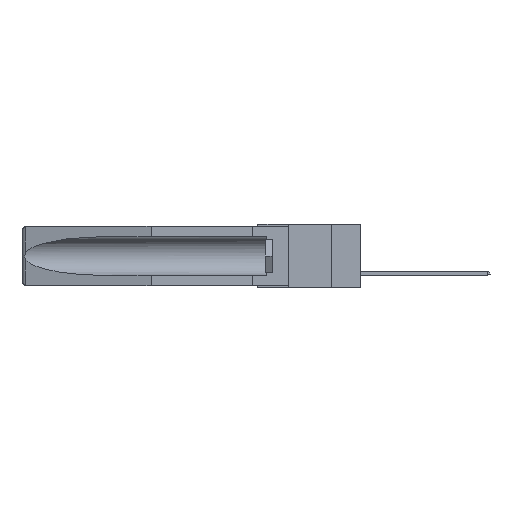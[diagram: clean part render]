
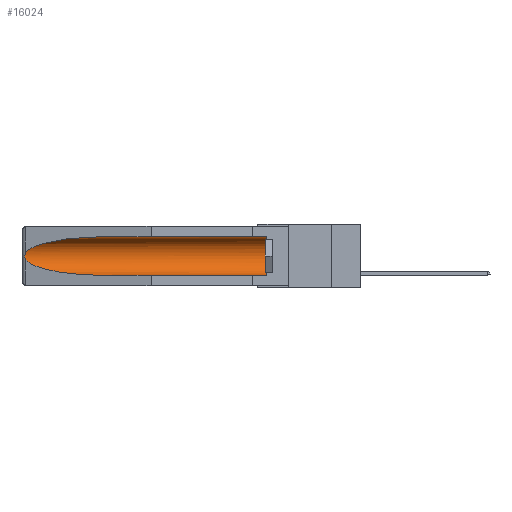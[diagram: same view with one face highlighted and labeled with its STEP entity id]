
A CAD part, left-side view. The second image highlights one B-rep face of the part: STEP entity #16024.
In plain terms, the highlighted cylindrical face has radius 2.857 mm (diameter 5.715 mm), a partial arc.
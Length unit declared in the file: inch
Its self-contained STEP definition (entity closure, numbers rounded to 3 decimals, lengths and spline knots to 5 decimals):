
#19 = CARTESIAN_POINT ( 'NONE',  ( 0.26537, 1.52718, -0.19328 ) ) ;
#266 = VERTEX_POINT ( 'NONE', #15615 ) ;
#373 = CARTESIAN_POINT ( 'NONE',  ( 0.155, 0.126, -0.284 ) ) ;
#1549 = VECTOR ( 'NONE', #12569, 39.37008 ) ;
#1816 = CARTESIAN_POINT ( 'NONE',  ( 0.21114, 1.30732, -0.059 ) ) ;
#2175 = CARTESIAN_POINT ( 'NONE',  ( 0.26537, 1.52718, -0.19328 ) ) ;
#2181 = DIRECTION ( 'NONE',  ( 0., -1., 0. ) ) ;
#2322 = ORIENTED_EDGE ( 'NONE', *, *, #21729, .T. ) ;
#2821 = CARTESIAN_POINT ( 'NONE',  ( 0.26537, 1.52718, -0.14972 ) ) ;
#2902 = EDGE_CURVE ( 'NONE', #9322, #266, #14139, .T. ) ;
#3323 = LINE ( 'NONE', #6932, #21889 ) ;
#3482 = CARTESIAN_POINT ( 'NONE',  ( 0.26537, 1.52718, -0.14972 ) ) ;
#3795 = DIRECTION ( 'NONE',  ( 0., 0., 1. ) ) ;
#3933 = CARTESIAN_POINT ( 'NONE',  ( 0.25451, 1.48313, -0.24835 ) ) ;
#4010 = CARTESIAN_POINT ( 'NONE',  ( 0.21114, 1.30732, -0.284 ) ) ;
#4280 = CARTESIAN_POINT ( 'NONE',  ( 0.155, 0.126, -0.1715 ) ) ;
#4368 = CARTESIAN_POINT ( 'NONE',  ( 0.2675, 1.53308, -0.17534 ) ) ;
#4770 = EDGE_CURVE ( 'NONE', #266, #13743, #3323, .T. ) ;
#5142 = CARTESIAN_POINT ( 'NONE',  ( 0.26537, 1.52718, -0.19328 ) ) ;
#5516 = DIRECTION ( 'NONE',  ( 0., 1., 0. ) ) ;
#5972 = EDGE_CURVE ( 'NONE', #9322, #6898, #13689, .T. ) ;
#6318 = CARTESIAN_POINT ( 'NONE',  ( 0.2673, 1.53269, -0.17917 ) ) ;
#6404 = CARTESIAN_POINT ( 'NONE',  ( 0.26597, 1.52961, -0.15275 ) ) ;
#6898 = VERTEX_POINT ( 'NONE', #12935 ) ;
#6932 = CARTESIAN_POINT ( 'NONE',  ( 0.155, -0.30754, -0.059 ) ) ;
#8266 = CARTESIAN_POINT ( 'NONE',  ( 0.2675, 1.53308, -0.16763 ) ) ;
#8625 = DIRECTION ( 'NONE',  ( 0., 1., 0. ) ) ;
#8796 = ORIENTED_EDGE ( 'NONE', *, *, #22874, .T. ) ;
#9172 = ORIENTED_EDGE ( 'NONE', *, *, #20537, .T. ) ;
#9322 = VERTEX_POINT ( 'NONE', #373 ) ;
#9352 =( BOUNDED_CURVE ( )  B_SPLINE_CURVE ( 3, ( #18686, #1816, #14677, #20545 ),
 .UNSPECIFIED., .F., .F. ) 
 B_SPLINE_CURVE_WITH_KNOTS ( ( 4, 4 ),
 ( 4.71239, 6.08839 ),
 .UNSPECIFIED. ) 
 CURVE ( )  GEOMETRIC_REPRESENTATION_ITEM ( )  RATIONAL_B_SPLINE_CURVE ( ( 1., 0.848, 0.848, 1. ) ) 
 REPRESENTATION_ITEM ( '' )  );
#11912 = VERTEX_POINT ( 'NONE', #3482 ) ;
#12319 =( BOUNDED_CURVE ( )  B_SPLINE_CURVE ( 3, ( #2175, #3933, #4010, #14855 ),
 .UNSPECIFIED., .F., .F. ) 
 B_SPLINE_CURVE_WITH_KNOTS ( ( 4, 4 ),
 ( 0.1948, 1.5708 ),
 .UNSPECIFIED. ) 
 CURVE ( )  GEOMETRIC_REPRESENTATION_ITEM ( )  RATIONAL_B_SPLINE_CURVE ( ( 1., 0.848, 0.848, 1. ) ) 
 REPRESENTATION_ITEM ( '' )  );
#12569 = DIRECTION ( 'NONE',  ( 0., 1., 0. ) ) ;
#12935 = CARTESIAN_POINT ( 'NONE',  ( 0.155, 1.07973, -0.284 ) ) ;
#13689 = LINE ( 'NONE', #23695, #1549 ) ;
#13743 = VERTEX_POINT ( 'NONE', #23746 ) ;
#13830 = VERTEX_POINT ( 'NONE', #19 ) ;
#13891 = AXIS2_PLACEMENT_3D ( 'NONE', #4280, #2181, #15032 ) ;
#14139 = CIRCLE ( 'NONE', #13891, 0.1125 ) ;
#14677 = CARTESIAN_POINT ( 'NONE',  ( 0.25451, 1.48313, -0.09465 ) ) ;
#14802 = CARTESIAN_POINT ( 'NONE',  ( 0.155, -0.30754, -0.1715 ) ) ;
#14855 = CARTESIAN_POINT ( 'NONE',  ( 0.155, 1.07973, -0.284 ) ) ;
#15032 = DIRECTION ( 'NONE',  ( 0., 0., 1. ) ) ;
#15446 = B_SPLINE_CURVE_WITH_KNOTS ( 'NONE', 3,
 ( #2821, #6404, #21553, #19383, #8266, #4368, #6318, #22184, #18811, #5142 ),
 .UNSPECIFIED., .F., .F.,
 ( 4, 2, 2, 2, 4 ),
 ( 0., 0.00029, 0.00058, 0.00087, 0.00117 ),
 .UNSPECIFIED. ) ;
#15615 = CARTESIAN_POINT ( 'NONE',  ( 0.155, 0.126, -0.059 ) ) ;
#16024 = ADVANCED_FACE ( 'NONE', ( #19517 ), #20105, .F. ) ;
#16887 = ORIENTED_EDGE ( 'NONE', *, *, #5972, .F. ) ;
#17447 = EDGE_LOOP ( 'NONE', ( #2322, #9172, #8796, #16887, #20429, #20836 ) ) ;
#18686 = CARTESIAN_POINT ( 'NONE',  ( 0.155, 1.07973, -0.059 ) ) ;
#18811 = CARTESIAN_POINT ( 'NONE',  ( 0.26597, 1.5296, -0.19026 ) ) ;
#19383 = CARTESIAN_POINT ( 'NONE',  ( 0.2673, 1.5327, -0.16383 ) ) ;
#19517 = FACE_OUTER_BOUND ( 'NONE', #17447, .T. ) ;
#20105 = CYLINDRICAL_SURFACE ( 'NONE', #21407, 0.1125 ) ;
#20429 = ORIENTED_EDGE ( 'NONE', *, *, #2902, .T. ) ;
#20537 = EDGE_CURVE ( 'NONE', #11912, #13830, #15446, .T. ) ;
#20545 = CARTESIAN_POINT ( 'NONE',  ( 0.26537, 1.52718, -0.14972 ) ) ;
#20836 = ORIENTED_EDGE ( 'NONE', *, *, #4770, .T. ) ;
#21407 = AXIS2_PLACEMENT_3D ( 'NONE', #14802, #5516, #3795 ) ;
#21553 = CARTESIAN_POINT ( 'NONE',  ( 0.26654, 1.53092, -0.15636 ) ) ;
#21729 = EDGE_CURVE ( 'NONE', #13743, #11912, #9352, .T. ) ;
#21889 = VECTOR ( 'NONE', #8625, 39.37008 ) ;
#22184 = CARTESIAN_POINT ( 'NONE',  ( 0.26655, 1.53094, -0.18657 ) ) ;
#22874 = EDGE_CURVE ( 'NONE', #13830, #6898, #12319, .T. ) ;
#23695 = CARTESIAN_POINT ( 'NONE',  ( 0.155, -0.30754, -0.284 ) ) ;
#23746 = CARTESIAN_POINT ( 'NONE',  ( 0.155, 1.07973, -0.059 ) ) ;
